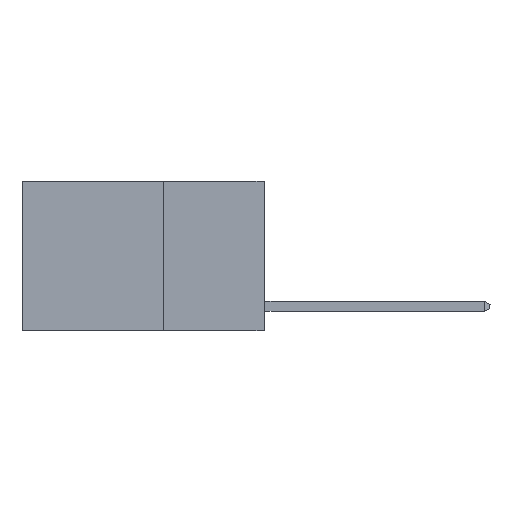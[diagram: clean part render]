
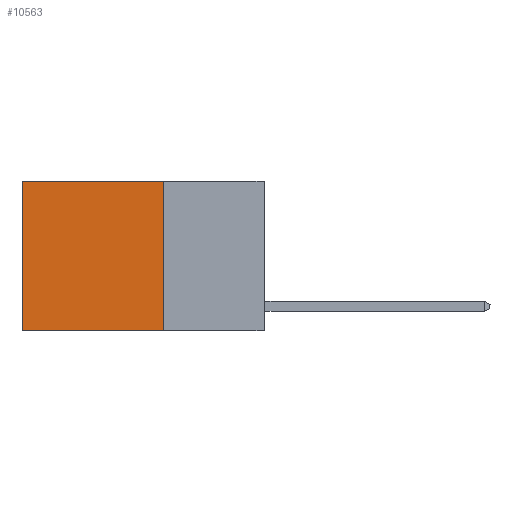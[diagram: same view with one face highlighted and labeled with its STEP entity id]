
A CAD part, left-side view. The second image highlights one B-rep face of the part: STEP entity #10563.
In plain terms, the highlighted planar face has unit normal (-1, 0, 0).
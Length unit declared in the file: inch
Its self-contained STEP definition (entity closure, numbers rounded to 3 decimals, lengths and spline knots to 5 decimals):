
#150 = LINE ( 'NONE', #17432, #4220 ) ;
#198 = EDGE_CURVE ( 'NONE', #11761, #6081, #15052, .T. ) ;
#1282 = PLANE ( 'NONE',  #18610 ) ;
#1512 = ORIENTED_EDGE ( 'NONE', *, *, #11054, .F. ) ;
#2688 = EDGE_CURVE ( 'NONE', #17955, #11761, #16292, .T. ) ;
#2785 = CARTESIAN_POINT ( 'NONE',  ( 0.2625, 0.25, 0. ) ) ;
#4220 = VECTOR ( 'NONE', #14515, 39.37008 ) ;
#4470 = EDGE_CURVE ( 'NONE', #10575, #6081, #9573, .T. ) ;
#4749 = ORIENTED_EDGE ( 'NONE', *, *, #198, .T. ) ;
#5594 = VECTOR ( 'NONE', #10006, 39.37008 ) ;
#5677 = FACE_OUTER_BOUND ( 'NONE', #13554, .T. ) ;
#5872 = CARTESIAN_POINT ( 'NONE',  ( 0.2625, 0.25, 0. ) ) ;
#6081 = VERTEX_POINT ( 'NONE', #10999 ) ;
#7358 = DIRECTION ( 'NONE',  ( 0., 0., -1. ) ) ;
#8089 = CARTESIAN_POINT ( 'NONE',  ( 0.2625, 0.6, 0. ) ) ;
#8440 = VECTOR ( 'NONE', #11867, 39.37008 ) ;
#9573 = LINE ( 'NONE', #14404, #5594 ) ;
#10006 = DIRECTION ( 'NONE',  ( 0., 1., 0. ) ) ;
#10563 = ADVANCED_FACE ( 'NONE', ( #5677 ), #1282, .F. ) ;
#10575 = VERTEX_POINT ( 'NONE', #19128 ) ;
#10999 = CARTESIAN_POINT ( 'NONE',  ( 0.2625, 0.6, -0.37 ) ) ;
#11054 = EDGE_CURVE ( 'NONE', #17955, #10575, #150, .T. ) ;
#11761 = VERTEX_POINT ( 'NONE', #11985 ) ;
#11867 = DIRECTION ( 'NONE',  ( 0., 1., 0. ) ) ;
#11985 = CARTESIAN_POINT ( 'NONE',  ( 0.2625, 0.6, 0. ) ) ;
#13554 = EDGE_LOOP ( 'NONE', ( #4749, #14629, #1512, #14264 ) ) ;
#13672 = CARTESIAN_POINT ( 'NONE',  ( 0.2625, 0.25, 0. ) ) ;
#14264 = ORIENTED_EDGE ( 'NONE', *, *, #2688, .T. ) ;
#14404 = CARTESIAN_POINT ( 'NONE',  ( 0.2625, 0.25, -0.37 ) ) ;
#14515 = DIRECTION ( 'NONE',  ( 0., 0., -1. ) ) ;
#14629 = ORIENTED_EDGE ( 'NONE', *, *, #4470, .F. ) ;
#15052 = LINE ( 'NONE', #8089, #18434 ) ;
#16220 = DIRECTION ( 'NONE',  ( 1., 0., 0. ) ) ;
#16292 = LINE ( 'NONE', #2785, #8440 ) ;
#16426 = DIRECTION ( 'NONE',  ( 0., 0., -1. ) ) ;
#17432 = CARTESIAN_POINT ( 'NONE',  ( 0.2625, 0.25, 0. ) ) ;
#17955 = VERTEX_POINT ( 'NONE', #13672 ) ;
#18434 = VECTOR ( 'NONE', #16426, 39.37008 ) ;
#18610 = AXIS2_PLACEMENT_3D ( 'NONE', #5872, #16220, #7358 ) ;
#19128 = CARTESIAN_POINT ( 'NONE',  ( 0.2625, 0.25, -0.37 ) ) ;
